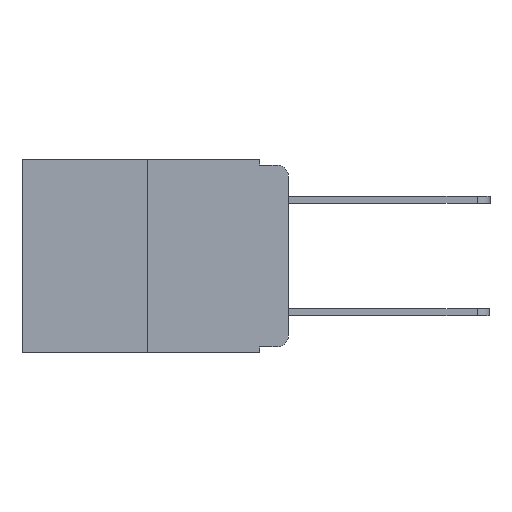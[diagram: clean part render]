
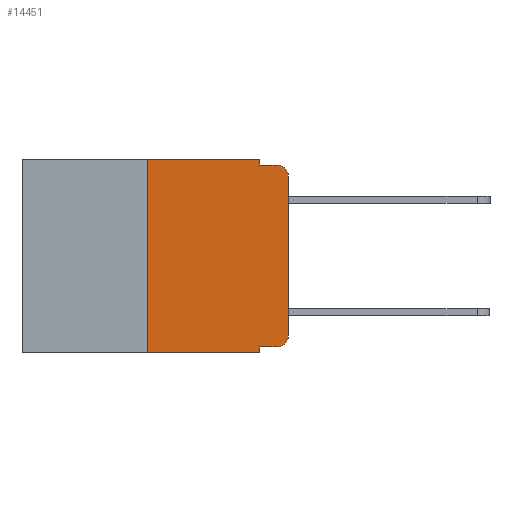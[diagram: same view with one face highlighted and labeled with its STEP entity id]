
A CAD part, left-side view. The second image highlights one B-rep face of the part: STEP entity #14451.
In plain terms, the highlighted planar face has unit normal (-1, 0, 0).
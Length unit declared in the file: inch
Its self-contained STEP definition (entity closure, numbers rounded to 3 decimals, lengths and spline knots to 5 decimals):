
#25 = LINE ( 'NONE', #909, #8089 ) ;
#198 = LINE ( 'NONE', #18607, #19074 ) ;
#615 = CARTESIAN_POINT ( 'NONE',  ( 0., 0.02, -0.01 ) ) ;
#827 = LINE ( 'NONE', #8278, #19156 ) ;
#909 = CARTESIAN_POINT ( 'NONE',  ( 0., 0.051, 0. ) ) ;
#1171 = ORIENTED_EDGE ( 'NONE', *, *, #10265, .T. ) ;
#2429 = EDGE_CURVE ( 'NONE', #13384, #17184, #6998, .T. ) ;
#2448 = CARTESIAN_POINT ( 'NONE',  ( 0., 0.473, 0. ) ) ;
#2760 = DIRECTION ( 'NONE',  ( 0., 0., -1. ) ) ;
#3335 = ORIENTED_EDGE ( 'NONE', *, *, #14970, .F. ) ;
#3423 = DIRECTION ( 'NONE',  ( 0., 0., 1. ) ) ;
#3425 = DIRECTION ( 'NONE',  ( 0., 0., 1. ) ) ;
#3538 = DIRECTION ( 'NONE',  ( 0., 0., -1. ) ) ;
#3705 = VERTEX_POINT ( 'NONE', #6200 ) ;
#3738 = DIRECTION ( 'NONE',  ( -1., 0., 0. ) ) ;
#3831 = VERTEX_POINT ( 'NONE', #615 ) ;
#4067 = VECTOR ( 'NONE', #3423, 39.37008 ) ;
#4075 = DIRECTION ( 'NONE',  ( 0., -1., 0. ) ) ;
#4219 = AXIS2_PLACEMENT_3D ( 'NONE', #5424, #15736, #7011 ) ;
#4325 = VERTEX_POINT ( 'NONE', #9751 ) ;
#4388 = FACE_OUTER_BOUND ( 'NONE', #5161, .T. ) ;
#4559 = CARTESIAN_POINT ( 'NONE',  ( 0., 0.02, -0.313 ) ) ;
#5161 = EDGE_LOOP ( 'NONE', ( #6259, #8444, #11625, #3335, #8181, #12545, #1171, #13885, #6986, #8902 ) ) ;
#5424 = CARTESIAN_POINT ( 'NONE',  ( 0., 0.02, -0.03 ) ) ;
#5452 = CARTESIAN_POINT ( 'NONE',  ( 0., 0., -0.313 ) ) ;
#6114 = EDGE_CURVE ( 'NONE', #17184, #12791, #12624, .T. ) ;
#6200 = CARTESIAN_POINT ( 'NONE',  ( 0., 0.051, -0.01 ) ) ;
#6250 = EDGE_CURVE ( 'NONE', #14999, #19219, #6345, .T. ) ;
#6259 = ORIENTED_EDGE ( 'NONE', *, *, #6114, .T. ) ;
#6345 = LINE ( 'NONE', #2448, #13740 ) ;
#6593 = VECTOR ( 'NONE', #3425, 39.37008 ) ;
#6986 = ORIENTED_EDGE ( 'NONE', *, *, #18605, .T. ) ;
#6998 = CIRCLE ( 'NONE', #13752, 0.02 ) ;
#7011 = DIRECTION ( 'NONE',  ( 0., 0., -1. ) ) ;
#7090 = LINE ( 'NONE', #15437, #6593 ) ;
#8089 = VECTOR ( 'NONE', #10423, 39.37008 ) ;
#8156 = EDGE_CURVE ( 'NONE', #12791, #3831, #12554, .T. ) ;
#8181 = ORIENTED_EDGE ( 'NONE', *, *, #6250, .F. ) ;
#8278 = CARTESIAN_POINT ( 'NONE',  ( 0., 0.473, -0.343 ) ) ;
#8444 = ORIENTED_EDGE ( 'NONE', *, *, #8156, .T. ) ;
#8689 = DIRECTION ( 'NONE',  ( 0., 0., -1. ) ) ;
#8902 = ORIENTED_EDGE ( 'NONE', *, *, #2429, .T. ) ;
#9296 = CARTESIAN_POINT ( 'NONE',  ( 0., 0.051, -0.333 ) ) ;
#9751 = CARTESIAN_POINT ( 'NONE',  ( 0., 0.051, -0.333 ) ) ;
#10183 = EDGE_CURVE ( 'NONE', #3705, #3831, #13595, .T. ) ;
#10265 = EDGE_CURVE ( 'NONE', #16527, #16041, #827, .T. ) ;
#10423 = DIRECTION ( 'NONE',  ( 0., 0., -1. ) ) ;
#10483 = CARTESIAN_POINT ( 'NONE',  ( 0., 0.25, 0. ) ) ;
#10612 = CARTESIAN_POINT ( 'NONE',  ( 0., 0.051, 0. ) ) ;
#10927 = CARTESIAN_POINT ( 'NONE',  ( 0., 0.02, -0.333 ) ) ;
#11625 = ORIENTED_EDGE ( 'NONE', *, *, #10183, .F. ) ;
#11961 = DIRECTION ( 'NONE',  ( 1., 0., 0. ) ) ;
#12503 = DIRECTION ( 'NONE',  ( 0., -1., 0. ) ) ;
#12545 = ORIENTED_EDGE ( 'NONE', *, *, #15907, .F. ) ;
#12554 = CIRCLE ( 'NONE', #4219, 0.02 ) ;
#12624 = LINE ( 'NONE', #16698, #4067 ) ;
#12688 = DIRECTION ( 'NONE',  ( 0., -1., 0. ) ) ;
#12791 = VERTEX_POINT ( 'NONE', #13903 ) ;
#13384 = VERTEX_POINT ( 'NONE', #10927 ) ;
#13595 = LINE ( 'NONE', #13946, #16854 ) ;
#13740 = VECTOR ( 'NONE', #4075, 39.37008 ) ;
#13752 = AXIS2_PLACEMENT_3D ( 'NONE', #4559, #3738, #3538 ) ;
#13885 = ORIENTED_EDGE ( 'NONE', *, *, #17722, .F. ) ;
#13903 = CARTESIAN_POINT ( 'NONE',  ( 0., 0., -0.03 ) ) ;
#13946 = CARTESIAN_POINT ( 'NONE',  ( 0., 0.051, -0.01 ) ) ;
#14315 = CARTESIAN_POINT ( 'NONE',  ( 0., 0.051, -0.343 ) ) ;
#14451 = ADVANCED_FACE ( 'NONE', ( #4388 ), #14775, .F. ) ;
#14775 = PLANE ( 'NONE',  #16367 ) ;
#14970 = EDGE_CURVE ( 'NONE', #19219, #3705, #25, .T. ) ;
#14999 = VERTEX_POINT ( 'NONE', #10483 ) ;
#15437 = CARTESIAN_POINT ( 'NONE',  ( 0., 0.25, 0. ) ) ;
#15736 = DIRECTION ( 'NONE',  ( -1., 0., 0. ) ) ;
#15840 = CARTESIAN_POINT ( 'NONE',  ( 0., 0.25, -0.343 ) ) ;
#15907 = EDGE_CURVE ( 'NONE', #16527, #14999, #7090, .T. ) ;
#16041 = VERTEX_POINT ( 'NONE', #14315 ) ;
#16367 = AXIS2_PLACEMENT_3D ( 'NONE', #18883, #11961, #2760 ) ;
#16430 = DIRECTION ( 'NONE',  ( 0., -1., 0. ) ) ;
#16527 = VERTEX_POINT ( 'NONE', #15840 ) ;
#16698 = CARTESIAN_POINT ( 'NONE',  ( 0., 0., 0. ) ) ;
#16854 = VECTOR ( 'NONE', #12503, 39.37008 ) ;
#17184 = VERTEX_POINT ( 'NONE', #5452 ) ;
#17722 = EDGE_CURVE ( 'NONE', #4325, #16041, #198, .T. ) ;
#18605 = EDGE_CURVE ( 'NONE', #4325, #13384, #19043, .T. ) ;
#18607 = CARTESIAN_POINT ( 'NONE',  ( 0., 0.051, 0. ) ) ;
#18858 = VECTOR ( 'NONE', #16430, 39.37008 ) ;
#18883 = CARTESIAN_POINT ( 'NONE',  ( 0., 0.473, 0. ) ) ;
#19043 = LINE ( 'NONE', #9296, #18858 ) ;
#19074 = VECTOR ( 'NONE', #8689, 39.37008 ) ;
#19156 = VECTOR ( 'NONE', #12688, 39.37008 ) ;
#19219 = VERTEX_POINT ( 'NONE', #10612 ) ;
